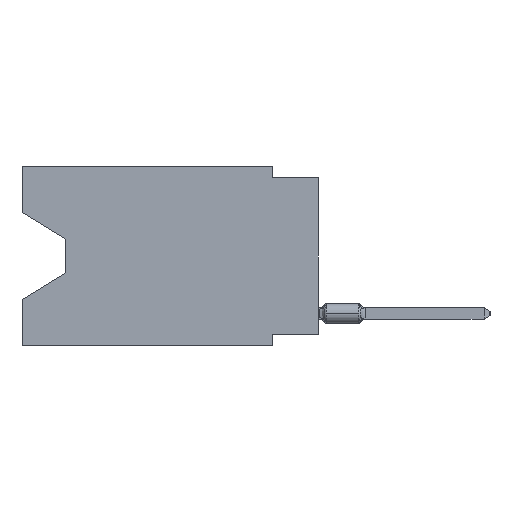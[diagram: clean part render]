
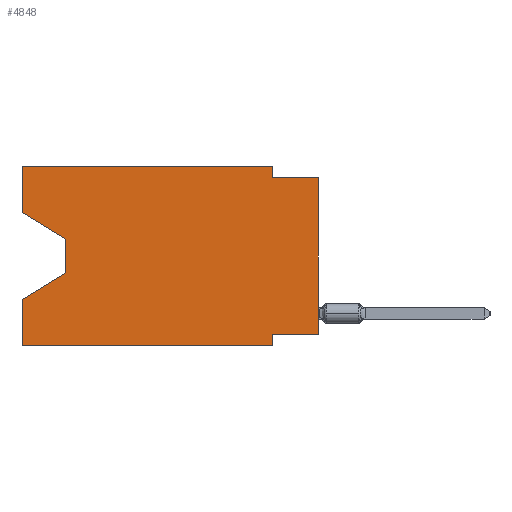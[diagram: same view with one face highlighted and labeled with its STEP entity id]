
A CAD part, left-side view. The second image highlights one B-rep face of the part: STEP entity #4848.
In plain terms, the highlighted planar face has unit normal (-1, 0, 0).
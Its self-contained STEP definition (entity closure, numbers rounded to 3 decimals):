
#537 = DIRECTION ( 'NONE',  ( 0., 1., 0. ) ) ;
#703 = VERTEX_POINT ( 'NONE', #2070 ) ;
#795 = VERTEX_POINT ( 'NONE', #15405 ) ;
#1098 = ORIENTED_EDGE ( 'NONE', *, *, #48253, .T. ) ;
#1467 = DIRECTION ( 'NONE',  ( 0., 0., 1. ) ) ;
#2070 = CARTESIAN_POINT ( 'NONE',  ( 0., 0., -0.635 ) ) ;
#4446 = LINE ( 'NONE', #29080, #26637 ) ;
#4558 = EDGE_CURVE ( 'NONE', #37492, #795, #62585, .T. ) ;
#4848 = ADVANCED_FACE ( 'NONE', ( #55652 ), #17649, .F. ) ;
#5232 = CARTESIAN_POINT ( 'NONE',  ( 0., 16.383, 0. ) ) ;
#8036 = DIRECTION ( 'NONE',  ( 0., 0., -1. ) ) ;
#8981 = VECTOR ( 'NONE', #62152, 1000. ) ;
#12354 = VERTEX_POINT ( 'NONE', #21538 ) ;
#13028 = ORIENTED_EDGE ( 'NONE', *, *, #38305, .T. ) ;
#13197 = LINE ( 'NONE', #13590, #20510 ) ;
#13590 = CARTESIAN_POINT ( 'NONE',  ( 0., 0., 0. ) ) ;
#14203 = VECTOR ( 'NONE', #24063, 1000. ) ;
#14259 = CARTESIAN_POINT ( 'NONE',  ( 0., 16.383, -9.906 ) ) ;
#14758 = ORIENTED_EDGE ( 'NONE', *, *, #64650, .T. ) ;
#15099 = ORIENTED_EDGE ( 'NONE', *, *, #60902, .T. ) ;
#15405 = CARTESIAN_POINT ( 'NONE',  ( 0., 2.54, -9.906 ) ) ;
#17649 = PLANE ( 'NONE',  #31181 ) ;
#18881 = LINE ( 'NONE', #79924, #8981 ) ;
#20510 = VECTOR ( 'NONE', #1467, 1000. ) ;
#20513 = DIRECTION ( 'NONE',  ( 0., 0., -1. ) ) ;
#20634 = CARTESIAN_POINT ( 'NONE',  ( 0., 16.383, 0. ) ) ;
#20754 = VECTOR ( 'NONE', #58631, 1000. ) ;
#21538 = CARTESIAN_POINT ( 'NONE',  ( 0., 13.97, -5.893 ) ) ;
#22946 = VERTEX_POINT ( 'NONE', #34106 ) ;
#23333 = EDGE_CURVE ( 'NONE', #12354, #28528, #58273, .T. ) ;
#23650 = ORIENTED_EDGE ( 'NONE', *, *, #23333, .T. ) ;
#23671 = CARTESIAN_POINT ( 'NONE',  ( 0., 2.54, 0. ) ) ;
#24063 = DIRECTION ( 'NONE',  ( 0., 0., -1. ) ) ;
#24403 = CARTESIAN_POINT ( 'NONE',  ( 0., 2.54, -9.271 ) ) ;
#26563 = EDGE_CURVE ( 'NONE', #64826, #28528, #4446, .T. ) ;
#26637 = VECTOR ( 'NONE', #53750, 1000. ) ;
#26723 = CARTESIAN_POINT ( 'NONE',  ( 0., 13.97, -5.893 ) ) ;
#26726 = VECTOR ( 'NONE', #71193, 1000. ) ;
#27886 = LINE ( 'NONE', #20634, #20754 ) ;
#28141 = ORIENTED_EDGE ( 'NONE', *, *, #64225, .F. ) ;
#28528 = VERTEX_POINT ( 'NONE', #42067 ) ;
#28704 = LINE ( 'NONE', #5232, #67297 ) ;
#29080 = CARTESIAN_POINT ( 'NONE',  ( 0., 16.383, 0. ) ) ;
#29695 = VECTOR ( 'NONE', #537, 1000. ) ;
#30621 = ORIENTED_EDGE ( 'NONE', *, *, #41696, .F. ) ;
#30841 = CARTESIAN_POINT ( 'NONE',  ( 0., 0., -9.271 ) ) ;
#30933 = LINE ( 'NONE', #23671, #14203 ) ;
#31181 = AXIS2_PLACEMENT_3D ( 'NONE', #41921, #43119, #37448 ) ;
#31204 = VERTEX_POINT ( 'NONE', #40434 ) ;
#31600 = EDGE_CURVE ( 'NONE', #56447, #64638, #30933, .T. ) ;
#33652 = LINE ( 'NONE', #14259, #60380 ) ;
#34106 = CARTESIAN_POINT ( 'NONE',  ( 0., 13.97, -4.013 ) ) ;
#35170 = DIRECTION ( 'NONE',  ( 0., 0., 1. ) ) ;
#37146 = VERTEX_POINT ( 'NONE', #44222 ) ;
#37448 = DIRECTION ( 'NONE',  ( 0., 0., -1. ) ) ;
#37492 = VERTEX_POINT ( 'NONE', #24403 ) ;
#38305 = EDGE_CURVE ( 'NONE', #37146, #703, #13197, .T. ) ;
#38720 = CARTESIAN_POINT ( 'NONE',  ( 0., 2.54, 0. ) ) ;
#40434 = CARTESIAN_POINT ( 'NONE',  ( 0., 16.383, -2.546 ) ) ;
#41014 = ORIENTED_EDGE ( 'NONE', *, *, #73873, .F. ) ;
#41225 = VECTOR ( 'NONE', #69045, 1000. ) ;
#41696 = EDGE_CURVE ( 'NONE', #50894, #56447, #27886, .T. ) ;
#41921 = CARTESIAN_POINT ( 'NONE',  ( 0., 16.383, 0. ) ) ;
#42067 = CARTESIAN_POINT ( 'NONE',  ( 0., 16.383, -7.36 ) ) ;
#42127 = EDGE_LOOP ( 'NONE', ( #14758, #1098, #23650, #72194, #15099, #79799, #41014, #13028, #28141, #55684, #30621, #46670 ) ) ;
#43119 = DIRECTION ( 'NONE',  ( 1., 0., 0. ) ) ;
#44107 = EDGE_CURVE ( 'NONE', #31204, #50894, #28704, .T. ) ;
#44222 = CARTESIAN_POINT ( 'NONE',  ( 0., 0., -9.271 ) ) ;
#44755 = CARTESIAN_POINT ( 'NONE',  ( 0., 16.383, -9.906 ) ) ;
#44791 = LINE ( 'NONE', #69454, #41225 ) ;
#45782 = DIRECTION ( 'NONE',  ( 0., -1., 0. ) ) ;
#46628 = VECTOR ( 'NONE', #8036, 1000. ) ;
#46670 = ORIENTED_EDGE ( 'NONE', *, *, #44107, .F. ) ;
#48253 = EDGE_CURVE ( 'NONE', #22946, #12354, #57307, .T. ) ;
#50461 = CARTESIAN_POINT ( 'NONE',  ( 0., 2.54, -9.906 ) ) ;
#50894 = VERTEX_POINT ( 'NONE', #56098 ) ;
#51235 = CARTESIAN_POINT ( 'NONE',  ( 0., 13.97, -4.013 ) ) ;
#51715 = VECTOR ( 'NONE', #20513, 1000. ) ;
#53750 = DIRECTION ( 'NONE',  ( 0., 0., 1. ) ) ;
#55652 = FACE_OUTER_BOUND ( 'NONE', #42127, .T. ) ;
#55684 = ORIENTED_EDGE ( 'NONE', *, *, #31600, .F. ) ;
#56098 = CARTESIAN_POINT ( 'NONE',  ( 0., 16.383, 0. ) ) ;
#56447 = VERTEX_POINT ( 'NONE', #38720 ) ;
#57307 = LINE ( 'NONE', #51235, #51715 ) ;
#58273 = LINE ( 'NONE', #26723, #26726 ) ;
#58631 = DIRECTION ( 'NONE',  ( 0., -1., 0. ) ) ;
#60380 = VECTOR ( 'NONE', #45782, 1000. ) ;
#60552 = CARTESIAN_POINT ( 'NONE',  ( 0., 2.54, -0.635 ) ) ;
#60902 = EDGE_CURVE ( 'NONE', #64826, #795, #33652, .T. ) ;
#61575 = LINE ( 'NONE', #30841, #29695 ) ;
#62152 = DIRECTION ( 'NONE',  ( 0., -0.855, -0.519 ) ) ;
#62585 = LINE ( 'NONE', #50461, #46628 ) ;
#64225 = EDGE_CURVE ( 'NONE', #64638, #703, #44791, .T. ) ;
#64638 = VERTEX_POINT ( 'NONE', #60552 ) ;
#64650 = EDGE_CURVE ( 'NONE', #31204, #22946, #18881, .T. ) ;
#64826 = VERTEX_POINT ( 'NONE', #44755 ) ;
#67297 = VECTOR ( 'NONE', #35170, 1000. ) ;
#69045 = DIRECTION ( 'NONE',  ( 0., -1., 0. ) ) ;
#69454 = CARTESIAN_POINT ( 'NONE',  ( 0., 0., -0.635 ) ) ;
#71193 = DIRECTION ( 'NONE',  ( 0., 0.855, -0.519 ) ) ;
#72194 = ORIENTED_EDGE ( 'NONE', *, *, #26563, .F. ) ;
#73873 = EDGE_CURVE ( 'NONE', #37146, #37492, #61575, .T. ) ;
#79799 = ORIENTED_EDGE ( 'NONE', *, *, #4558, .F. ) ;
#79924 = CARTESIAN_POINT ( 'NONE',  ( 0., 16.383, -2.546 ) ) ;
